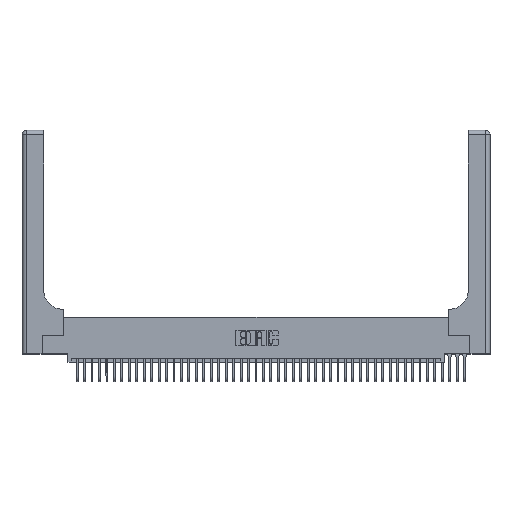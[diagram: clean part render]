
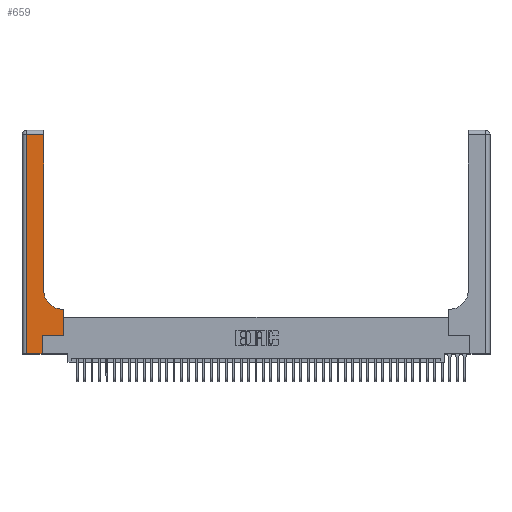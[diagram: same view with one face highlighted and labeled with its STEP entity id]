
A CAD part, top view. The second image highlights one B-rep face of the part: STEP entity #659.
In plain terms, the highlighted planar face has unit normal (0, 0, 1).
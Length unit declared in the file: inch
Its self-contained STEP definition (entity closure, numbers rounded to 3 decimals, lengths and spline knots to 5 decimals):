
#656 = DIRECTION ( 'NONE',  ( 1., 0., 0. ) ) ;
#659 = ADVANCED_FACE ( 'NONE', ( #14769 ), #13479, .F. ) ;
#1189 = AXIS2_PLACEMENT_3D ( 'NONE', #35483, #38548, #20014 ) ;
#1496 = CARTESIAN_POINT ( 'NONE',  ( 0.5415, 0.85, 0.37 ) ) ;
#1903 = VECTOR ( 'NONE', #2053, 39.37008 ) ;
#1920 = DIRECTION ( 'NONE',  ( 1., 0., 0. ) ) ;
#2053 = DIRECTION ( 'NONE',  ( 0., 1., 0. ) ) ;
#4030 = ORIENTED_EDGE ( 'NONE', *, *, #8597, .T. ) ;
#4036 = VECTOR ( 'NONE', #22036, 39.37008 ) ;
#4902 = DIRECTION ( 'NONE',  ( 1., 0., 0. ) ) ;
#5993 = EDGE_CURVE ( 'NONE', #7977, #14106, #16922, .T. ) ;
#6869 = DIRECTION ( 'NONE',  ( -1., 0., 0. ) ) ;
#6982 = AXIS2_PLACEMENT_3D ( 'NONE', #1496, #24468, #4902 ) ;
#7426 = DIRECTION ( 'NONE',  ( -1., 0., 0. ) ) ;
#7544 = CARTESIAN_POINT ( 'NONE',  ( 0.5415, 0.6, 0.37 ) ) ;
#7746 = EDGE_CURVE ( 'NONE', #17640, #36604, #13036, .T. ) ;
#7913 = LINE ( 'NONE', #40116, #15766 ) ;
#7977 = VERTEX_POINT ( 'NONE', #38900 ) ;
#8227 = EDGE_LOOP ( 'NONE', ( #16561, #14059, #20701, #4030, #37560, #23444, #34875, #32120, #33439 ) ) ;
#8231 = EDGE_CURVE ( 'NONE', #39483, #9032, #10872, .T. ) ;
#8597 = EDGE_CURVE ( 'NONE', #36604, #7977, #21540, .T. ) ;
#9032 = VERTEX_POINT ( 'NONE', #25880 ) ;
#10152 = CARTESIAN_POINT ( 'NONE',  ( 0.06, 2.94, 0.37 ) ) ;
#10872 = LINE ( 'NONE', #21847, #1903 ) ;
#11830 = EDGE_CURVE ( 'NONE', #18169, #19799, #7913, .T. ) ;
#13036 = LINE ( 'NONE', #25028, #4036 ) ;
#13479 = PLANE ( 'NONE',  #1189 ) ;
#14059 = ORIENTED_EDGE ( 'NONE', *, *, #15884, .T. ) ;
#14106 = VERTEX_POINT ( 'NONE', #34985 ) ;
#14769 = FACE_OUTER_BOUND ( 'NONE', #8227, .T. ) ;
#15766 = VECTOR ( 'NONE', #37042, 39.37008 ) ;
#15792 = VECTOR ( 'NONE', #6869, 39.37008 ) ;
#15884 = EDGE_CURVE ( 'NONE', #19799, #17640, #27160, .T. ) ;
#16046 = CARTESIAN_POINT ( 'NONE',  ( 0.2915, 0.85, 0.37 ) ) ;
#16560 = LINE ( 'NONE', #23681, #23001 ) ;
#16561 = ORIENTED_EDGE ( 'NONE', *, *, #11830, .T. ) ;
#16728 = VECTOR ( 'NONE', #1920, 39.37008 ) ;
#16922 = LINE ( 'NONE', #37455, #39796 ) ;
#17640 = VERTEX_POINT ( 'NONE', #10152 ) ;
#18169 = VERTEX_POINT ( 'NONE', #16046 ) ;
#18427 = CARTESIAN_POINT ( 'NONE',  ( 0.2915, 2.94, 0.37 ) ) ;
#18485 = VERTEX_POINT ( 'NONE', #7544 ) ;
#19799 = VERTEX_POINT ( 'NONE', #18427 ) ;
#20014 = DIRECTION ( 'NONE',  ( -1., 0., 0. ) ) ;
#20589 = CARTESIAN_POINT ( 'NONE',  ( 0., 0., 0.37 ) ) ;
#20701 = ORIENTED_EDGE ( 'NONE', *, *, #7746, .T. ) ;
#21540 = LINE ( 'NONE', #20589, #22516 ) ;
#21847 = CARTESIAN_POINT ( 'NONE',  ( 0.5585, 0.25, 0.37 ) ) ;
#22036 = DIRECTION ( 'NONE',  ( 0., -1., 0. ) ) ;
#22516 = VECTOR ( 'NONE', #656, 39.37008 ) ;
#23001 = VECTOR ( 'NONE', #7426, 39.37008 ) ;
#23142 = CARTESIAN_POINT ( 'NONE',  ( 0., 2.94, 0.37 ) ) ;
#23444 = ORIENTED_EDGE ( 'NONE', *, *, #27999, .T. ) ;
#23681 = CARTESIAN_POINT ( 'NONE',  ( 0.2915, 0.6, 0.37 ) ) ;
#24468 = DIRECTION ( 'NONE',  ( 0., 0., -1. ) ) ;
#25028 = CARTESIAN_POINT ( 'NONE',  ( 0.06, 3., 0.37 ) ) ;
#25138 = LINE ( 'NONE', #30965, #16728 ) ;
#25880 = CARTESIAN_POINT ( 'NONE',  ( 0.5585, 0.6, 0.37 ) ) ;
#26620 = CIRCLE ( 'NONE', #6982, 0.25 ) ;
#27160 = LINE ( 'NONE', #23142, #15792 ) ;
#27999 = EDGE_CURVE ( 'NONE', #14106, #39483, #25138, .T. ) ;
#29348 = CARTESIAN_POINT ( 'NONE',  ( 0.5585, 0.25, 0.37 ) ) ;
#30965 = CARTESIAN_POINT ( 'NONE',  ( 0.269, 0.25, 0.37 ) ) ;
#32120 = ORIENTED_EDGE ( 'NONE', *, *, #36414, .T. ) ;
#33439 = ORIENTED_EDGE ( 'NONE', *, *, #39103, .T. ) ;
#33794 = CARTESIAN_POINT ( 'NONE',  ( 0.06, 0., 0.37 ) ) ;
#34875 = ORIENTED_EDGE ( 'NONE', *, *, #8231, .T. ) ;
#34985 = CARTESIAN_POINT ( 'NONE',  ( 0.269, 0.25, 0.37 ) ) ;
#35483 = CARTESIAN_POINT ( 'NONE',  ( 0., 3., 0.37 ) ) ;
#36414 = EDGE_CURVE ( 'NONE', #9032, #18485, #16560, .T. ) ;
#36604 = VERTEX_POINT ( 'NONE', #33794 ) ;
#37042 = DIRECTION ( 'NONE',  ( 0., 1., 0. ) ) ;
#37455 = CARTESIAN_POINT ( 'NONE',  ( 0.269, 0., 0.37 ) ) ;
#37560 = ORIENTED_EDGE ( 'NONE', *, *, #5993, .T. ) ;
#38548 = DIRECTION ( 'NONE',  ( 0., 0., -1. ) ) ;
#38900 = CARTESIAN_POINT ( 'NONE',  ( 0.269, 0., 0.37 ) ) ;
#39103 = EDGE_CURVE ( 'NONE', #18485, #18169, #26620, .T. ) ;
#39483 = VERTEX_POINT ( 'NONE', #29348 ) ;
#39796 = VECTOR ( 'NONE', #40373, 39.37008 ) ;
#40116 = CARTESIAN_POINT ( 'NONE',  ( 0.2915, 3., 0.37 ) ) ;
#40373 = DIRECTION ( 'NONE',  ( 0., 1., 0. ) ) ;
